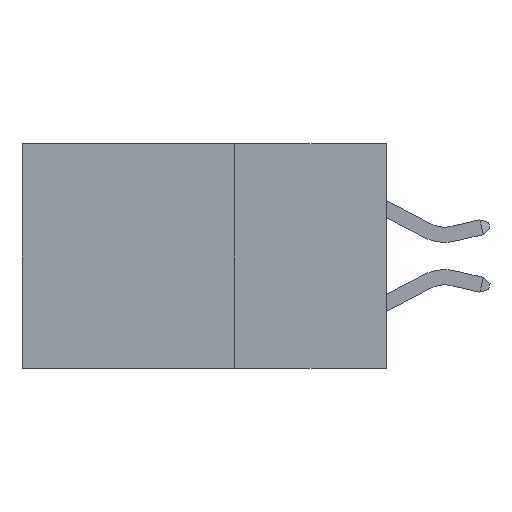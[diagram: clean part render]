
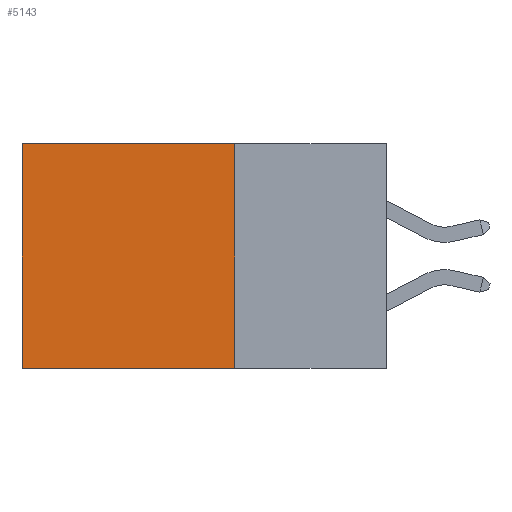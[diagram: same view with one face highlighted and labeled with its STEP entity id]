
A CAD part, left-side view. The second image highlights one B-rep face of the part: STEP entity #5143.
In plain terms, the highlighted planar face has unit normal (-1, 0, 0).
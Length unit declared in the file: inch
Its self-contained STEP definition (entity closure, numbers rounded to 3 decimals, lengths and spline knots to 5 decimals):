
#115 = EDGE_CURVE ( 'NONE', #14408, #7276, #6268, .T. ) ;
#310 = EDGE_CURVE ( 'NONE', #13271, #14408, #11934, .T. ) ;
#469 = EDGE_CURVE ( 'NONE', #13271, #2087, #3532, .T. ) ;
#1331 = FACE_OUTER_BOUND ( 'NONE', #2887, .T. ) ;
#2087 = VERTEX_POINT ( 'NONE', #13985 ) ;
#2887 = EDGE_LOOP ( 'NONE', ( #10880, #11229, #11318, #11660 ) ) ;
#3532 = LINE ( 'NONE', #7801, #9638 ) ;
#3564 = DIRECTION ( 'NONE',  ( 0., 0., -1. ) ) ;
#4087 = CARTESIAN_POINT ( 'NONE',  ( 0.2615, 0.25, -0.37 ) ) ;
#4281 = DIRECTION ( 'NONE',  ( 0., 0., -1. ) ) ;
#4286 = DIRECTION ( 'NONE',  ( 1., 0., 0. ) ) ;
#4307 = VECTOR ( 'NONE', #11434, 39.37008 ) ;
#4313 = CARTESIAN_POINT ( 'NONE',  ( 0.2615, 0.25, -0.37 ) ) ;
#4330 = PLANE ( 'NONE',  #9230 ) ;
#4721 = DIRECTION ( 'NONE',  ( 0., 1., 0. ) ) ;
#5143 = ADVANCED_FACE ( 'NONE', ( #1331 ), #4330, .F. ) ;
#5272 = CARTESIAN_POINT ( 'NONE',  ( 0.2615, 0.25, -0.37 ) ) ;
#5848 = EDGE_CURVE ( 'NONE', #2087, #7276, #10400, .T. ) ;
#6268 = LINE ( 'NONE', #6689, #14400 ) ;
#6689 = CARTESIAN_POINT ( 'NONE',  ( 0.2615, 0.25, -0.37 ) ) ;
#7276 = VERTEX_POINT ( 'NONE', #12004 ) ;
#7801 = CARTESIAN_POINT ( 'NONE',  ( 0.2615, 0.25, 0. ) ) ;
#8794 = CARTESIAN_POINT ( 'NONE',  ( 0.2615, 0.25, 0. ) ) ;
#9230 = AXIS2_PLACEMENT_3D ( 'NONE', #4313, #4286, #4281 ) ;
#9638 = VECTOR ( 'NONE', #4721, 39.37008 ) ;
#10400 = LINE ( 'NONE', #11584, #4307 ) ;
#10880 = ORIENTED_EDGE ( 'NONE', *, *, #5848, .T. ) ;
#11229 = ORIENTED_EDGE ( 'NONE', *, *, #115, .F. ) ;
#11318 = ORIENTED_EDGE ( 'NONE', *, *, #310, .F. ) ;
#11434 = DIRECTION ( 'NONE',  ( 0., 0., -1. ) ) ;
#11576 = VECTOR ( 'NONE', #3564, 39.37008 ) ;
#11584 = CARTESIAN_POINT ( 'NONE',  ( 0.2615, 0.6, -0.37 ) ) ;
#11660 = ORIENTED_EDGE ( 'NONE', *, *, #469, .T. ) ;
#11934 = LINE ( 'NONE', #5272, #11576 ) ;
#12004 = CARTESIAN_POINT ( 'NONE',  ( 0.2615, 0.6, -0.37 ) ) ;
#12183 = DIRECTION ( 'NONE',  ( 0., 1., 0. ) ) ;
#13271 = VERTEX_POINT ( 'NONE', #8794 ) ;
#13985 = CARTESIAN_POINT ( 'NONE',  ( 0.2615, 0.6, 0. ) ) ;
#14400 = VECTOR ( 'NONE', #12183, 39.37008 ) ;
#14408 = VERTEX_POINT ( 'NONE', #4087 ) ;
